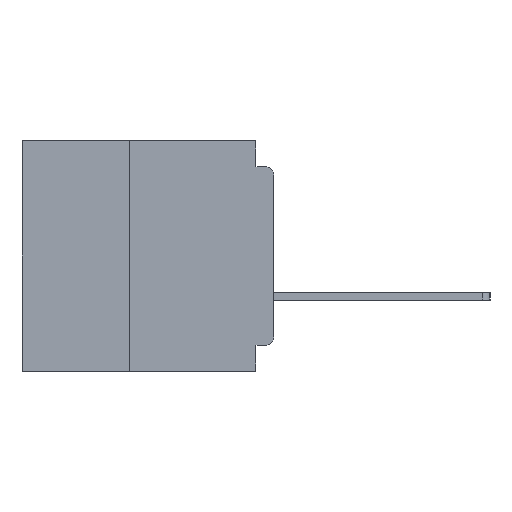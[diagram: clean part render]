
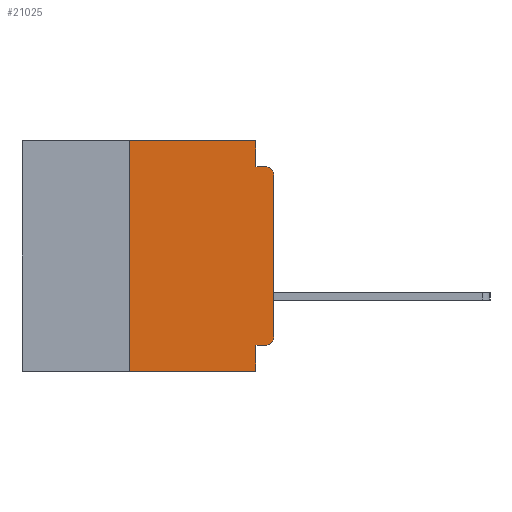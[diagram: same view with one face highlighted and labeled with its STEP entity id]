
A CAD part, left-side view. The second image highlights one B-rep face of the part: STEP entity #21025.
In plain terms, the highlighted planar face has unit normal (-1, 0, 0).
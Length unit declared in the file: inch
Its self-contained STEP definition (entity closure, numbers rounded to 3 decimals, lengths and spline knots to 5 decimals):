
#3 = ORIENTED_EDGE ( 'NONE', *, *, #1929, .F. ) ;
#239 = DIRECTION ( 'NONE',  ( 0., 0., -1. ) ) ;
#833 = DIRECTION ( 'NONE',  ( 0., 0., -1. ) ) ;
#986 = DIRECTION ( 'NONE',  ( -1., 0., 0. ) ) ;
#1873 = DIRECTION ( 'NONE',  ( 0., 0., 1. ) ) ;
#1929 = EDGE_CURVE ( 'NONE', #41418, #30476, #16479, .T. ) ;
#2034 = ORIENTED_EDGE ( 'NONE', *, *, #27237, .F. ) ;
#2379 = CARTESIAN_POINT ( 'NONE',  ( 0., 0.031, -0.045 ) ) ;
#2685 = DIRECTION ( 'NONE',  ( 0., 0., 1. ) ) ;
#3335 = CARTESIAN_POINT ( 'NONE',  ( 0., 0., -0.045 ) ) ;
#3516 = EDGE_CURVE ( 'NONE', #19235, #39154, #19284, .T. ) ;
#3758 = LINE ( 'NONE', #11775, #29837 ) ;
#4329 = ORIENTED_EDGE ( 'NONE', *, *, #3516, .F. ) ;
#4569 = AXIS2_PLACEMENT_3D ( 'NONE', #17297, #20572, #833 ) ;
#4694 = CARTESIAN_POINT ( 'NONE',  ( 0., 0.031, -0.4 ) ) ;
#4911 = EDGE_CURVE ( 'NONE', #29893, #30476, #40888, .T. ) ;
#5193 = CARTESIAN_POINT ( 'NONE',  ( 0., 0., -0.06 ) ) ;
#6357 = DIRECTION ( 'NONE',  ( 0., 0., -1. ) ) ;
#6903 = EDGE_CURVE ( 'NONE', #23922, #41418, #27690, .T. ) ;
#7035 = CARTESIAN_POINT ( 'NONE',  ( 0., 0., -0.34 ) ) ;
#8396 = CARTESIAN_POINT ( 'NONE',  ( 0., 0.015, -0.045 ) ) ;
#8776 = CARTESIAN_POINT ( 'NONE',  ( 0., 0., 0. ) ) ;
#8821 = VECTOR ( 'NONE', #2685, 39.37008 ) ;
#9796 = VECTOR ( 'NONE', #24804, 39.37008 ) ;
#9810 = ORIENTED_EDGE ( 'NONE', *, *, #33325, .T. ) ;
#10794 = DIRECTION ( 'NONE',  ( 0., -1., 0. ) ) ;
#11353 = ORIENTED_EDGE ( 'NONE', *, *, #12196, .T. ) ;
#11775 = CARTESIAN_POINT ( 'NONE',  ( 0., 0.437, 0. ) ) ;
#12196 = EDGE_CURVE ( 'NONE', #34235, #39920, #20907, .T. ) ;
#12598 = VERTEX_POINT ( 'NONE', #13014 ) ;
#13014 = CARTESIAN_POINT ( 'NONE',  ( 0., 0.25, -0.4 ) ) ;
#14395 = ORIENTED_EDGE ( 'NONE', *, *, #4911, .T. ) ;
#16064 = AXIS2_PLACEMENT_3D ( 'NONE', #39326, #19973, #239 ) ;
#16479 = LINE ( 'NONE', #3335, #41271 ) ;
#17297 = CARTESIAN_POINT ( 'NONE',  ( 0., 0.437, 0. ) ) ;
#17711 = CARTESIAN_POINT ( 'NONE',  ( 0., 0.015, -0.355 ) ) ;
#18442 = LINE ( 'NONE', #37598, #9796 ) ;
#19043 = VECTOR ( 'NONE', #33825, 39.37008 ) ;
#19235 = VERTEX_POINT ( 'NONE', #22353 ) ;
#19284 = LINE ( 'NONE', #19379, #35409 ) ;
#19379 = CARTESIAN_POINT ( 'NONE',  ( 0., 0.031, -0.4 ) ) ;
#19950 = LINE ( 'NONE', #8776, #36087 ) ;
#19973 = DIRECTION ( 'NONE',  ( -1., 0., 0. ) ) ;
#20539 = AXIS2_PLACEMENT_3D ( 'NONE', #20730, #986, #23981 ) ;
#20572 = DIRECTION ( 'NONE',  ( 1., 0., 0. ) ) ;
#20730 = CARTESIAN_POINT ( 'NONE',  ( 0., 0.015, -0.34 ) ) ;
#20812 = ORIENTED_EDGE ( 'NONE', *, *, #31340, .T. ) ;
#20907 = CIRCLE ( 'NONE', #20539, 0.015 ) ;
#21025 = ADVANCED_FACE ( 'NONE', ( #34013 ), #36638, .F. ) ;
#21106 = EDGE_LOOP ( 'NONE', ( #9810, #14395, #3, #37110, #25612, #29853, #20812, #4329, #2034, #11353 ) ) ;
#22353 = CARTESIAN_POINT ( 'NONE',  ( 0., 0.031, -0.355 ) ) ;
#23922 = VERTEX_POINT ( 'NONE', #36579 ) ;
#23981 = DIRECTION ( 'NONE',  ( 0., 0., -1. ) ) ;
#24744 = EDGE_CURVE ( 'NONE', #31316, #23922, #3758, .T. ) ;
#24804 = DIRECTION ( 'NONE',  ( 0., 1., 0. ) ) ;
#25612 = ORIENTED_EDGE ( 'NONE', *, *, #24744, .F. ) ;
#27237 = EDGE_CURVE ( 'NONE', #34235, #19235, #18442, .T. ) ;
#27690 = LINE ( 'NONE', #30617, #19043 ) ;
#29837 = VECTOR ( 'NONE', #37516, 39.37008 ) ;
#29853 = ORIENTED_EDGE ( 'NONE', *, *, #38790, .F. ) ;
#29893 = VERTEX_POINT ( 'NONE', #5193 ) ;
#30234 = CARTESIAN_POINT ( 'NONE',  ( 0., 0.437, -0.4 ) ) ;
#30476 = VERTEX_POINT ( 'NONE', #8396 ) ;
#30617 = CARTESIAN_POINT ( 'NONE',  ( 0., 0.031, 0. ) ) ;
#30708 = VECTOR ( 'NONE', #10794, 39.37008 ) ;
#31316 = VERTEX_POINT ( 'NONE', #33038 ) ;
#31340 = EDGE_CURVE ( 'NONE', #12598, #39154, #31712, .T. ) ;
#31712 = LINE ( 'NONE', #30234, #30708 ) ;
#33038 = CARTESIAN_POINT ( 'NONE',  ( 0., 0.25, 0. ) ) ;
#33325 = EDGE_CURVE ( 'NONE', #39920, #29893, #19950, .T. ) ;
#33825 = DIRECTION ( 'NONE',  ( 0., 0., -1. ) ) ;
#34013 = FACE_OUTER_BOUND ( 'NONE', #21106, .T. ) ;
#34235 = VERTEX_POINT ( 'NONE', #17711 ) ;
#34654 = LINE ( 'NONE', #41696, #8821 ) ;
#35409 = VECTOR ( 'NONE', #6357, 39.37008 ) ;
#36087 = VECTOR ( 'NONE', #1873, 39.37008 ) ;
#36579 = CARTESIAN_POINT ( 'NONE',  ( 0., 0.031, 0. ) ) ;
#36638 = PLANE ( 'NONE',  #4569 ) ;
#37110 = ORIENTED_EDGE ( 'NONE', *, *, #6903, .F. ) ;
#37516 = DIRECTION ( 'NONE',  ( 0., -1., 0. ) ) ;
#37598 = CARTESIAN_POINT ( 'NONE',  ( 0., 0., -0.355 ) ) ;
#38790 = EDGE_CURVE ( 'NONE', #12598, #31316, #34654, .T. ) ;
#39048 = DIRECTION ( 'NONE',  ( 0., -1., 0. ) ) ;
#39154 = VERTEX_POINT ( 'NONE', #4694 ) ;
#39326 = CARTESIAN_POINT ( 'NONE',  ( 0., 0.015, -0.06 ) ) ;
#39920 = VERTEX_POINT ( 'NONE', #7035 ) ;
#40888 = CIRCLE ( 'NONE', #16064, 0.015 ) ;
#41271 = VECTOR ( 'NONE', #39048, 39.37008 ) ;
#41418 = VERTEX_POINT ( 'NONE', #2379 ) ;
#41696 = CARTESIAN_POINT ( 'NONE',  ( 0., 0.25, -0.4 ) ) ;
